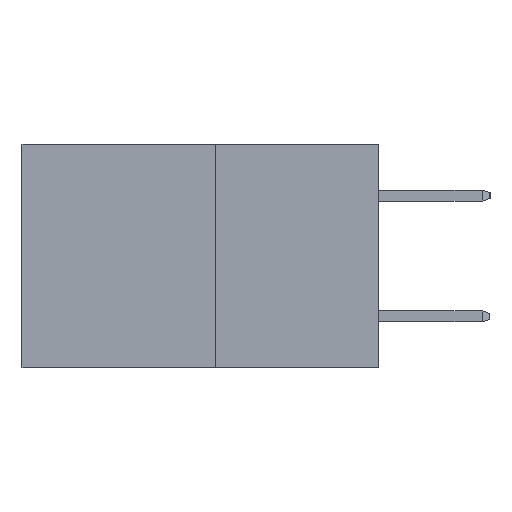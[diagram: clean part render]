
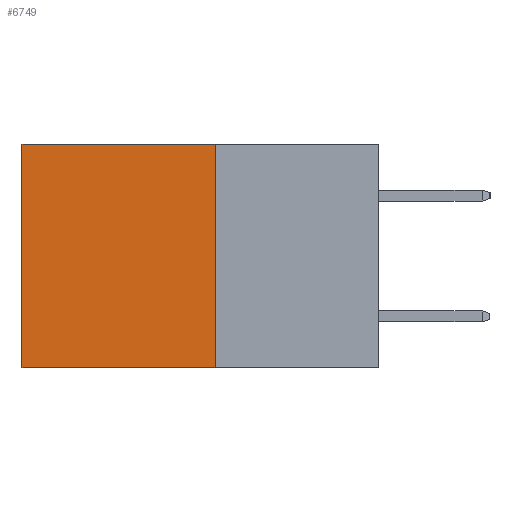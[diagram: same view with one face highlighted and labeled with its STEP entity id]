
A CAD part, left-side view. The second image highlights one B-rep face of the part: STEP entity #6749.
In plain terms, the highlighted planar face has unit normal (-1, 0, 0).
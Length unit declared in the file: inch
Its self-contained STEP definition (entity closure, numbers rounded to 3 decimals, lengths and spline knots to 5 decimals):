
#387 = LINE ( 'NONE', #4239, #8903 ) ;
#497 = DIRECTION ( 'NONE',  ( 0., 0., -1. ) ) ;
#689 = ORIENTED_EDGE ( 'NONE', *, *, #8864, .T. ) ;
#699 = ORIENTED_EDGE ( 'NONE', *, *, #3069, .F. ) ;
#759 = VERTEX_POINT ( 'NONE', #6896 ) ;
#766 = CARTESIAN_POINT ( 'NONE',  ( 0.277, 0.27, 0. ) ) ;
#883 = VECTOR ( 'NONE', #2684, 39.37008 ) ;
#897 = DIRECTION ( 'NONE',  ( 0., 0., -1. ) ) ;
#1235 = CARTESIAN_POINT ( 'NONE',  ( 0.277, 0.27, -0.37 ) ) ;
#1573 = ORIENTED_EDGE ( 'NONE', *, *, #7447, .F. ) ;
#1576 = DIRECTION ( 'NONE',  ( 0., 1., 0. ) ) ;
#1706 = VECTOR ( 'NONE', #497, 39.37008 ) ;
#1801 = CARTESIAN_POINT ( 'NONE',  ( 0.277, 0.59, 0. ) ) ;
#2102 = AXIS2_PLACEMENT_3D ( 'NONE', #7137, #9440, #4589 ) ;
#2161 = VERTEX_POINT ( 'NONE', #1801 ) ;
#2551 = ORIENTED_EDGE ( 'NONE', *, *, #7166, .T. ) ;
#2684 = DIRECTION ( 'NONE',  ( 0., 1., 0. ) ) ;
#3069 = EDGE_CURVE ( 'NONE', #3655, #759, #7592, .T. ) ;
#3655 = VERTEX_POINT ( 'NONE', #1235 ) ;
#4113 = VERTEX_POINT ( 'NONE', #766 ) ;
#4239 = CARTESIAN_POINT ( 'NONE',  ( 0.277, 0.59, -0.37 ) ) ;
#4587 = VECTOR ( 'NONE', #1576, 39.37008 ) ;
#4589 = DIRECTION ( 'NONE',  ( 0., 0., -1. ) ) ;
#5207 = FACE_OUTER_BOUND ( 'NONE', #5237, .T. ) ;
#5237 = EDGE_LOOP ( 'NONE', ( #689, #699, #1573, #2551 ) ) ;
#6715 = LINE ( 'NONE', #10231, #1706 ) ;
#6749 = ADVANCED_FACE ( 'NONE', ( #5207 ), #8674, .F. ) ;
#6865 = LINE ( 'NONE', #9712, #4587 ) ;
#6896 = CARTESIAN_POINT ( 'NONE',  ( 0.277, 0.59, -0.37 ) ) ;
#7137 = CARTESIAN_POINT ( 'NONE',  ( 0.277, 0.27, -0.37 ) ) ;
#7166 = EDGE_CURVE ( 'NONE', #4113, #2161, #6865, .T. ) ;
#7447 = EDGE_CURVE ( 'NONE', #4113, #3655, #6715, .T. ) ;
#7592 = LINE ( 'NONE', #7805, #883 ) ;
#7805 = CARTESIAN_POINT ( 'NONE',  ( 0.277, 0.27, -0.37 ) ) ;
#8674 = PLANE ( 'NONE',  #2102 ) ;
#8864 = EDGE_CURVE ( 'NONE', #2161, #759, #387, .T. ) ;
#8903 = VECTOR ( 'NONE', #897, 39.37008 ) ;
#9440 = DIRECTION ( 'NONE',  ( 1., 0., 0. ) ) ;
#9712 = CARTESIAN_POINT ( 'NONE',  ( 0.277, 0.27, 0. ) ) ;
#10231 = CARTESIAN_POINT ( 'NONE',  ( 0.277, 0.27, -0.37 ) ) ;
